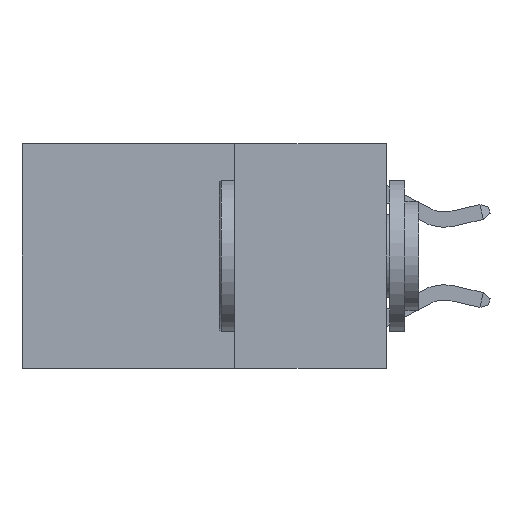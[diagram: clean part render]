
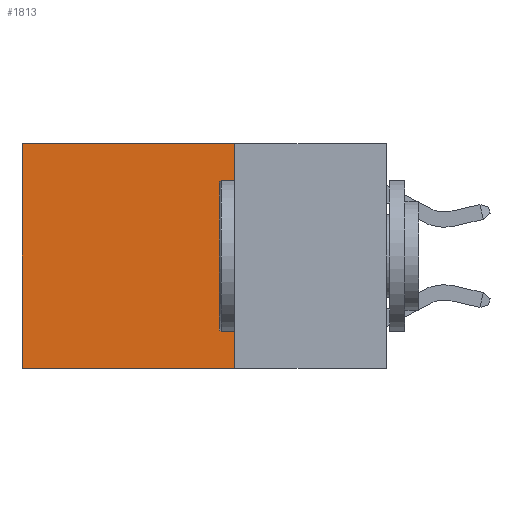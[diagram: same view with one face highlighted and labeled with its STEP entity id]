
A CAD part, left-side view. The second image highlights one B-rep face of the part: STEP entity #1813.
In plain terms, the highlighted planar face has unit normal (-1, 0, 0).
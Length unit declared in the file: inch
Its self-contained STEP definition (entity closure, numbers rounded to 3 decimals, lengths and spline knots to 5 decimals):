
#700 = LINE ( 'NONE', #2404, #816 ) ;
#816 = VECTOR ( 'NONE', #9830, 39.37008 ) ;
#947 = VERTEX_POINT ( 'NONE', #3869 ) ;
#1375 = LINE ( 'NONE', #21378, #6604 ) ;
#1813 = ADVANCED_FACE ( 'NONE', ( #8199 ), #21274, .F. ) ;
#2404 = CARTESIAN_POINT ( 'NONE',  ( 0.2625, 0.25, 0. ) ) ;
#2489 = CARTESIAN_POINT ( 'NONE',  ( 0.2625, 0.25, 0. ) ) ;
#2605 = LINE ( 'NONE', #2489, #3395 ) ;
#3395 = VECTOR ( 'NONE', #22846, 39.37008 ) ;
#3869 = CARTESIAN_POINT ( 'NONE',  ( 0.2625, 0.25, -0.37 ) ) ;
#4550 = DIRECTION ( 'NONE',  ( 1., 0., 0. ) ) ;
#6121 = EDGE_CURVE ( 'NONE', #23004, #11612, #11730, .T. ) ;
#6491 = DIRECTION ( 'NONE',  ( 0., 0., -1. ) ) ;
#6604 = VECTOR ( 'NONE', #19913, 39.37008 ) ;
#6776 = AXIS2_PLACEMENT_3D ( 'NONE', #10283, #4550, #6491 ) ;
#7286 = CARTESIAN_POINT ( 'NONE',  ( 0.2625, 0.25, 0. ) ) ;
#7433 = ORIENTED_EDGE ( 'NONE', *, *, #6121, .T. ) ;
#7451 = ORIENTED_EDGE ( 'NONE', *, *, #18638, .T. ) ;
#8199 = FACE_OUTER_BOUND ( 'NONE', #23489, .T. ) ;
#8668 = CARTESIAN_POINT ( 'NONE',  ( 0.2625, 0.6, 0. ) ) ;
#9830 = DIRECTION ( 'NONE',  ( 0., 1., 0. ) ) ;
#10283 = CARTESIAN_POINT ( 'NONE',  ( 0.2625, 0.25, 0. ) ) ;
#10608 = CARTESIAN_POINT ( 'NONE',  ( 0.2625, 0.6, -0.37 ) ) ;
#10765 = EDGE_CURVE ( 'NONE', #15684, #947, #2605, .T. ) ;
#11612 = VERTEX_POINT ( 'NONE', #10608 ) ;
#11730 = LINE ( 'NONE', #13671, #15503 ) ;
#13324 = DIRECTION ( 'NONE',  ( 0., 0., -1. ) ) ;
#13406 = EDGE_CURVE ( 'NONE', #947, #11612, #1375, .T. ) ;
#13671 = CARTESIAN_POINT ( 'NONE',  ( 0.2625, 0.6, 0. ) ) ;
#15503 = VECTOR ( 'NONE', #13324, 39.37008 ) ;
#15684 = VERTEX_POINT ( 'NONE', #7286 ) ;
#18638 = EDGE_CURVE ( 'NONE', #15684, #23004, #700, .T. ) ;
#19682 = ORIENTED_EDGE ( 'NONE', *, *, #13406, .F. ) ;
#19828 = ORIENTED_EDGE ( 'NONE', *, *, #10765, .F. ) ;
#19913 = DIRECTION ( 'NONE',  ( 0., 1., 0. ) ) ;
#21274 = PLANE ( 'NONE',  #6776 ) ;
#21378 = CARTESIAN_POINT ( 'NONE',  ( 0.2625, 0.25, -0.37 ) ) ;
#22846 = DIRECTION ( 'NONE',  ( 0., 0., -1. ) ) ;
#23004 = VERTEX_POINT ( 'NONE', #8668 ) ;
#23489 = EDGE_LOOP ( 'NONE', ( #7433, #19682, #19828, #7451 ) ) ;
